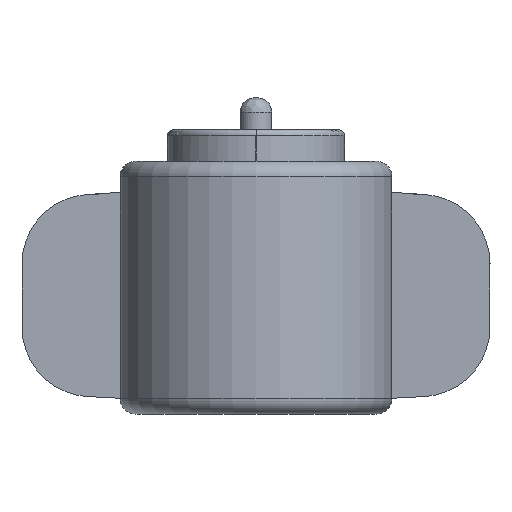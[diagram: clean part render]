
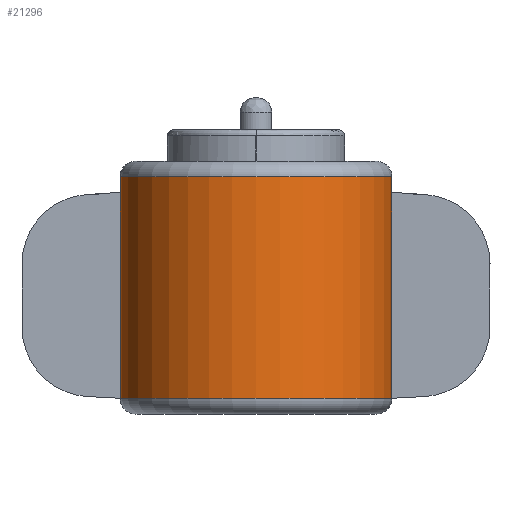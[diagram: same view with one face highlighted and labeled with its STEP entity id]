
A CAD part, left-side view. The second image highlights one B-rep face of the part: STEP entity #21296.
In plain terms, the highlighted cylindrical face has radius 4.3 mm (diameter 8.6 mm), a partial arc.
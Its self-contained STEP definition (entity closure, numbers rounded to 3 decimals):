
#1947 = CIRCLE ( 'NONE', #17359, 4.3 ) ;
#2226 = ORIENTED_EDGE ( 'NONE', *, *, #16596, .T. ) ;
#2277 = AXIS2_PLACEMENT_3D ( 'NONE', #10339, #8798, #13627 ) ;
#3279 = DIRECTION ( 'NONE',  ( 0., 1., 0. ) ) ;
#4094 = VERTEX_POINT ( 'NONE', #13266 ) ;
#4216 = DIRECTION ( 'NONE',  ( 0., 0., 1. ) ) ;
#5863 = FACE_OUTER_BOUND ( 'NONE', #18643, .T. ) ;
#7073 = DIRECTION ( 'NONE',  ( 0., 0., 1. ) ) ;
#8210 = LINE ( 'NONE', #10081, #11291 ) ;
#8798 = DIRECTION ( 'NONE',  ( 0., 0., -1. ) ) ;
#9233 = DIRECTION ( 'NONE',  ( 0., 0., -1. ) ) ;
#10035 = CARTESIAN_POINT ( 'NONE',  ( -8.63, -4.3, 0.5 ) ) ;
#10081 = CARTESIAN_POINT ( 'NONE',  ( -8.63, 4.3, -6.5 ) ) ;
#10339 = CARTESIAN_POINT ( 'NONE',  ( -8.63, 0., 0.5 ) ) ;
#10793 = VERTEX_POINT ( 'NONE', #13269 ) ;
#10812 = CYLINDRICAL_SURFACE ( 'NONE', #17818, 4.3 ) ;
#10994 = ORIENTED_EDGE ( 'NONE', *, *, #17190, .F. ) ;
#11291 = VECTOR ( 'NONE', #14691, 1000. ) ;
#11589 = VERTEX_POINT ( 'NONE', #12167 ) ;
#12167 = CARTESIAN_POINT ( 'NONE',  ( -8.63, -4.3, 0.5 ) ) ;
#13211 = DIRECTION ( 'NONE',  ( 1., 0., 0. ) ) ;
#13266 = CARTESIAN_POINT ( 'NONE',  ( -8.63, 4.3, 0.5 ) ) ;
#13269 = CARTESIAN_POINT ( 'NONE',  ( -8.63, 4.3, -6.5 ) ) ;
#13462 = CARTESIAN_POINT ( 'NONE',  ( -8.63, 0., -6.5 ) ) ;
#13627 = DIRECTION ( 'NONE',  ( -1., 0., 0. ) ) ;
#14602 = EDGE_CURVE ( 'NONE', #10793, #4094, #8210, .T. ) ;
#14691 = DIRECTION ( 'NONE',  ( 0., 0., 1. ) ) ;
#14810 = ORIENTED_EDGE ( 'NONE', *, *, #14602, .F. ) ;
#16118 = EDGE_CURVE ( 'NONE', #11589, #4094, #17678, .T. ) ;
#16596 = EDGE_CURVE ( 'NONE', #10793, #16758, #1947, .T. ) ;
#16615 = LINE ( 'NONE', #10035, #18063 ) ;
#16758 = VERTEX_POINT ( 'NONE', #19186 ) ;
#17190 = EDGE_CURVE ( 'NONE', #11589, #16758, #16615, .T. ) ;
#17359 = AXIS2_PLACEMENT_3D ( 'NONE', #13462, #7073, #3279 ) ;
#17504 = CARTESIAN_POINT ( 'NONE',  ( -8.63, 0., -6.64 ) ) ;
#17678 = CIRCLE ( 'NONE', #2277, 4.3 ) ;
#17818 = AXIS2_PLACEMENT_3D ( 'NONE', #17504, #4216, #13211 ) ;
#18063 = VECTOR ( 'NONE', #9233, 1000. ) ;
#18643 = EDGE_LOOP ( 'NONE', ( #10994, #19263, #14810, #2226 ) ) ;
#19186 = CARTESIAN_POINT ( 'NONE',  ( -8.63, -4.3, -6.5 ) ) ;
#19263 = ORIENTED_EDGE ( 'NONE', *, *, #16118, .T. ) ;
#21296 = ADVANCED_FACE ( 'NONE', ( #5863 ), #10812, .T. ) ;
